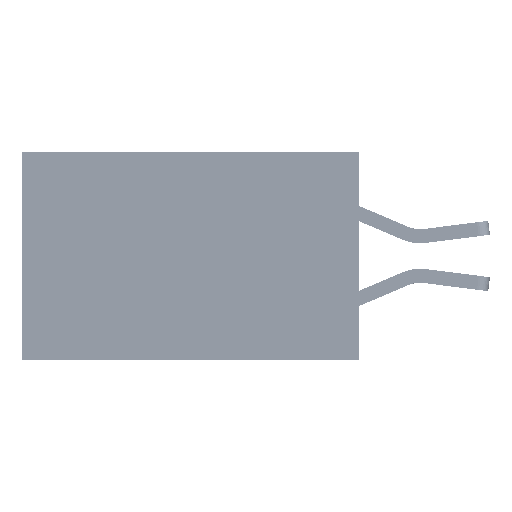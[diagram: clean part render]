
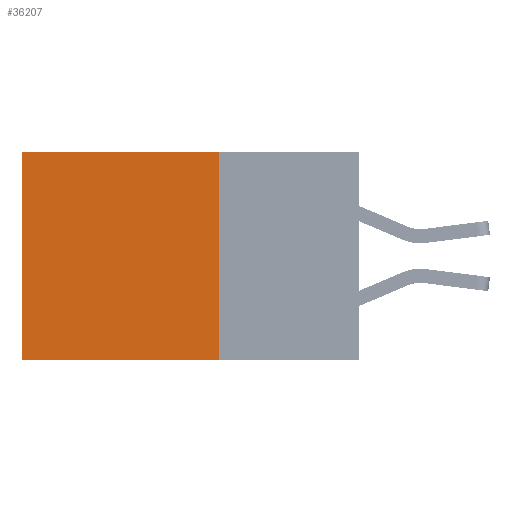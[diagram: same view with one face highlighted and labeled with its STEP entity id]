
A CAD part, left-side view. The second image highlights one B-rep face of the part: STEP entity #36207.
In plain terms, the highlighted planar face has unit normal (-1, 0, 0).
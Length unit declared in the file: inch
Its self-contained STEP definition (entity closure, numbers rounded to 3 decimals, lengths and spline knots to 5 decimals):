
#744 = LINE ( 'NONE', #32313, #33555 ) ;
#995 = VERTEX_POINT ( 'NONE', #8363 ) ;
#2605 = CARTESIAN_POINT ( 'NONE',  ( 0.2875, 0.6, 0. ) ) ;
#3023 = ORIENTED_EDGE ( 'NONE', *, *, #20773, .F. ) ;
#4845 = ORIENTED_EDGE ( 'NONE', *, *, #23069, .T. ) ;
#5288 = CARTESIAN_POINT ( 'NONE',  ( 0.2875, 0.6, -0.37 ) ) ;
#5600 = VECTOR ( 'NONE', #41399, 39.37008 ) ;
#5975 = DIRECTION ( 'NONE',  ( 0., 0., -1. ) ) ;
#6322 = DIRECTION ( 'NONE',  ( 0., 0., -1. ) ) ;
#8363 = CARTESIAN_POINT ( 'NONE',  ( 0.2875, 0.25, -0.37 ) ) ;
#9515 = DIRECTION ( 'NONE',  ( 1., 0., 0. ) ) ;
#10408 = DIRECTION ( 'NONE',  ( 0., 0., -1. ) ) ;
#11714 = EDGE_CURVE ( 'NONE', #29615, #995, #744, .T. ) ;
#11868 = VECTOR ( 'NONE', #6322, 39.37008 ) ;
#18436 = VECTOR ( 'NONE', #47004, 39.37008 ) ;
#20773 = EDGE_CURVE ( 'NONE', #995, #26526, #36898, .T. ) ;
#23069 = EDGE_CURVE ( 'NONE', #29615, #24755, #44698, .T. ) ;
#24755 = VERTEX_POINT ( 'NONE', #35631 ) ;
#26118 = ORIENTED_EDGE ( 'NONE', *, *, #11714, .F. ) ;
#26526 = VERTEX_POINT ( 'NONE', #5288 ) ;
#27684 = ORIENTED_EDGE ( 'NONE', *, *, #42493, .T. ) ;
#29615 = VERTEX_POINT ( 'NONE', #46384 ) ;
#31408 = PLANE ( 'NONE',  #32029 ) ;
#32029 = AXIS2_PLACEMENT_3D ( 'NONE', #38611, #9515, #5975 ) ;
#32313 = CARTESIAN_POINT ( 'NONE',  ( 0.2875, 0.25, 0. ) ) ;
#32860 = CARTESIAN_POINT ( 'NONE',  ( 0.2875, 0.25, -0.37 ) ) ;
#33555 = VECTOR ( 'NONE', #10408, 39.37008 ) ;
#35631 = CARTESIAN_POINT ( 'NONE',  ( 0.2875, 0.6, 0. ) ) ;
#36207 = ADVANCED_FACE ( 'NONE', ( #43396 ), #31408, .F. ) ;
#36898 = LINE ( 'NONE', #32860, #18436 ) ;
#38611 = CARTESIAN_POINT ( 'NONE',  ( 0.2875, 0.25, 0. ) ) ;
#40161 = EDGE_LOOP ( 'NONE', ( #27684, #3023, #26118, #4845 ) ) ;
#41399 = DIRECTION ( 'NONE',  ( 0., 1., 0. ) ) ;
#42493 = EDGE_CURVE ( 'NONE', #24755, #26526, #44059, .T. ) ;
#43396 = FACE_OUTER_BOUND ( 'NONE', #40161, .T. ) ;
#44059 = LINE ( 'NONE', #2605, #11868 ) ;
#44630 = CARTESIAN_POINT ( 'NONE',  ( 0.2875, 0.25, 0. ) ) ;
#44698 = LINE ( 'NONE', #44630, #5600 ) ;
#46384 = CARTESIAN_POINT ( 'NONE',  ( 0.2875, 0.25, 0. ) ) ;
#47004 = DIRECTION ( 'NONE',  ( 0., 1., 0. ) ) ;
